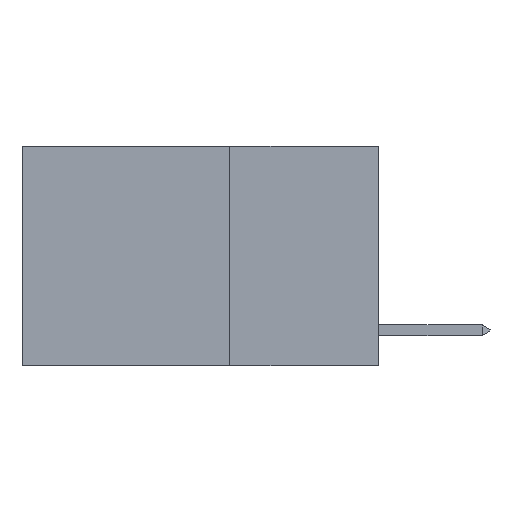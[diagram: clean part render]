
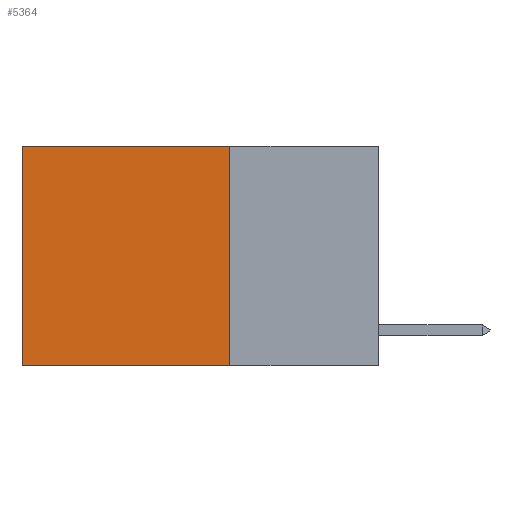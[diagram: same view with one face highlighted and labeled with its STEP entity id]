
A CAD part, left-side view. The second image highlights one B-rep face of the part: STEP entity #5364.
In plain terms, the highlighted planar face has unit normal (-1, 0, 0).
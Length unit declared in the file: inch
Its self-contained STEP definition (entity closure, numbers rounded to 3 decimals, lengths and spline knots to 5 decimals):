
#611 = LINE ( 'NONE', #3597, #1696 ) ;
#737 = VECTOR ( 'NONE', #4512, 39.37008 ) ;
#1376 = DIRECTION ( 'NONE',  ( 0., 0., -1. ) ) ;
#1696 = VECTOR ( 'NONE', #16894, 39.37008 ) ;
#2040 = ORIENTED_EDGE ( 'NONE', *, *, #17418, .T. ) ;
#2093 = EDGE_LOOP ( 'NONE', ( #2040, #3467, #8811, #3475 ) ) ;
#2907 = CARTESIAN_POINT ( 'NONE',  ( 0.2625, 0.25, 0. ) ) ;
#3467 = ORIENTED_EDGE ( 'NONE', *, *, #18034, .F. ) ;
#3475 = ORIENTED_EDGE ( 'NONE', *, *, #8638, .T. ) ;
#3597 = CARTESIAN_POINT ( 'NONE',  ( 0.2625, 0.25, -0.37 ) ) ;
#4014 = FACE_OUTER_BOUND ( 'NONE', #2093, .T. ) ;
#4147 = CARTESIAN_POINT ( 'NONE',  ( 0.2625, 0.25, 0. ) ) ;
#4445 = EDGE_CURVE ( 'NONE', #14856, #4587, #7339, .T. ) ;
#4512 = DIRECTION ( 'NONE',  ( 0., 0., -1. ) ) ;
#4587 = VERTEX_POINT ( 'NONE', #11581 ) ;
#5364 = ADVANCED_FACE ( 'NONE', ( #4014 ), #5588, .F. ) ;
#5588 = PLANE ( 'NONE',  #7564 ) ;
#6975 = VECTOR ( 'NONE', #7032, 39.37008 ) ;
#7032 = DIRECTION ( 'NONE',  ( 0., 1., 0. ) ) ;
#7339 = LINE ( 'NONE', #4147, #7535 ) ;
#7535 = VECTOR ( 'NONE', #1376, 39.37008 ) ;
#7564 = AXIS2_PLACEMENT_3D ( 'NONE', #16217, #7688, #16808 ) ;
#7688 = DIRECTION ( 'NONE',  ( 1., 0., 0. ) ) ;
#7970 = VERTEX_POINT ( 'NONE', #13841 ) ;
#8598 = CARTESIAN_POINT ( 'NONE',  ( 0.2625, 0.6, 0. ) ) ;
#8638 = EDGE_CURVE ( 'NONE', #14856, #7970, #13282, .T. ) ;
#8811 = ORIENTED_EDGE ( 'NONE', *, *, #4445, .F. ) ;
#9791 = CARTESIAN_POINT ( 'NONE',  ( 0.2625, 0.6, -0.37 ) ) ;
#11581 = CARTESIAN_POINT ( 'NONE',  ( 0.2625, 0.25, -0.37 ) ) ;
#13282 = LINE ( 'NONE', #19316, #6975 ) ;
#13738 = VERTEX_POINT ( 'NONE', #9791 ) ;
#13841 = CARTESIAN_POINT ( 'NONE',  ( 0.2625, 0.6, 0. ) ) ;
#14856 = VERTEX_POINT ( 'NONE', #2907 ) ;
#16217 = CARTESIAN_POINT ( 'NONE',  ( 0.2625, 0.25, 0. ) ) ;
#16808 = DIRECTION ( 'NONE',  ( 0., 0., -1. ) ) ;
#16894 = DIRECTION ( 'NONE',  ( 0., 1., 0. ) ) ;
#17418 = EDGE_CURVE ( 'NONE', #7970, #13738, #17626, .T. ) ;
#17626 = LINE ( 'NONE', #8598, #737 ) ;
#18034 = EDGE_CURVE ( 'NONE', #4587, #13738, #611, .T. ) ;
#19316 = CARTESIAN_POINT ( 'NONE',  ( 0.2625, 0.25, 0. ) ) ;
